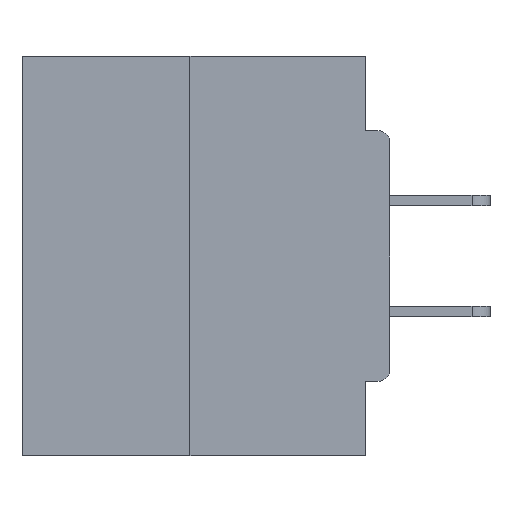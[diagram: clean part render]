
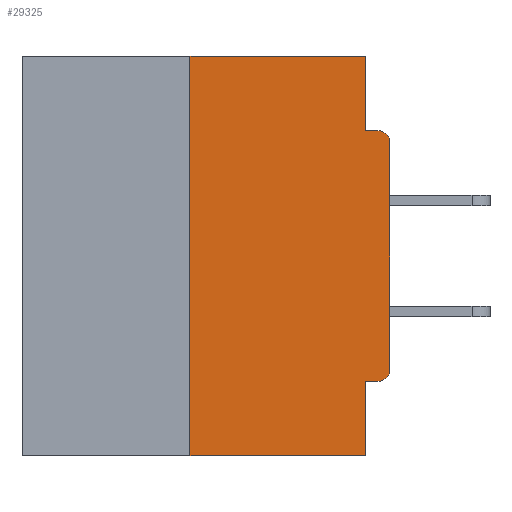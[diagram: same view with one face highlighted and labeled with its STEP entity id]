
A CAD part, left-side view. The second image highlights one B-rep face of the part: STEP entity #29325.
In plain terms, the highlighted planar face has unit normal (-1, 0, 0).
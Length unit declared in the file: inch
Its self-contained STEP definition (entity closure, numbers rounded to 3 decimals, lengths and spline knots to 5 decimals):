
#575 = LINE ( 'NONE', #21977, #9507 ) ;
#872 = CIRCLE ( 'NONE', #31588, 0.015 ) ;
#994 = CARTESIAN_POINT ( 'NONE',  ( 0., 0.46, 0. ) ) ;
#1197 = CARTESIAN_POINT ( 'NONE',  ( 0., 0.031, -0.0935 ) ) ;
#1281 = VECTOR ( 'NONE', #32515, 39.37008 ) ;
#1293 = CARTESIAN_POINT ( 'NONE',  ( 0., 0., -0.4065 ) ) ;
#1433 = DIRECTION ( 'NONE',  ( 0., -1., 0. ) ) ;
#2229 = LINE ( 'NONE', #38369, #1281 ) ;
#2484 = CARTESIAN_POINT ( 'NONE',  ( 0., 0., -0.3915 ) ) ;
#3401 = CARTESIAN_POINT ( 'NONE',  ( 0., 0.25, 0. ) ) ;
#3453 = VECTOR ( 'NONE', #20346, 39.37008 ) ;
#3644 = AXIS2_PLACEMENT_3D ( 'NONE', #15115, #14986, #6227 ) ;
#3993 = AXIS2_PLACEMENT_3D ( 'NONE', #36569, #6404, #12547 ) ;
#4587 = ORIENTED_EDGE ( 'NONE', *, *, #15984, .T. ) ;
#4954 = VECTOR ( 'NONE', #37236, 39.37008 ) ;
#5242 = DIRECTION ( 'NONE',  ( -1., 0., 0. ) ) ;
#6227 = DIRECTION ( 'NONE',  ( 0., 0., -1. ) ) ;
#6404 = DIRECTION ( 'NONE',  ( -1., 0., 0. ) ) ;
#7098 = VECTOR ( 'NONE', #31059, 39.37008 ) ;
#8372 = CARTESIAN_POINT ( 'NONE',  ( 0., 0.25, -0.5 ) ) ;
#8419 = VERTEX_POINT ( 'NONE', #30548 ) ;
#8903 = CARTESIAN_POINT ( 'NONE',  ( 0., 0.031, 0. ) ) ;
#9379 = EDGE_CURVE ( 'NONE', #21108, #22341, #33854, .T. ) ;
#9507 = VECTOR ( 'NONE', #12649, 39.37008 ) ;
#11661 = CARTESIAN_POINT ( 'NONE',  ( 0., 0.015, -0.1085 ) ) ;
#11968 = LINE ( 'NONE', #1293, #4954 ) ;
#12340 = LINE ( 'NONE', #22180, #3453 ) ;
#12547 = DIRECTION ( 'NONE',  ( 0., 0., -1. ) ) ;
#12649 = DIRECTION ( 'NONE',  ( 0., 0., 1. ) ) ;
#12778 = ORIENTED_EDGE ( 'NONE', *, *, #9379, .F. ) ;
#14009 = CARTESIAN_POINT ( 'NONE',  ( 0., 0., -0.1085 ) ) ;
#14609 = ORIENTED_EDGE ( 'NONE', *, *, #23510, .T. ) ;
#14707 = CARTESIAN_POINT ( 'NONE',  ( 0., 0.25, 0. ) ) ;
#14986 = DIRECTION ( 'NONE',  ( 1., 0., 0. ) ) ;
#15112 = ORIENTED_EDGE ( 'NONE', *, *, #18907, .F. ) ;
#15115 = CARTESIAN_POINT ( 'NONE',  ( 0., 0.46, 0. ) ) ;
#15802 = ORIENTED_EDGE ( 'NONE', *, *, #32103, .F. ) ;
#15984 = EDGE_CURVE ( 'NONE', #31399, #33786, #575, .T. ) ;
#16483 = VECTOR ( 'NONE', #29881, 39.37008 ) ;
#18907 = EDGE_CURVE ( 'NONE', #22341, #27713, #22138, .T. ) ;
#18994 = FACE_OUTER_BOUND ( 'NONE', #32371, .T. ) ;
#19898 = VERTEX_POINT ( 'NONE', #8372 ) ;
#20346 = DIRECTION ( 'NONE',  ( 0., -1., 0. ) ) ;
#20741 = CARTESIAN_POINT ( 'NONE',  ( 0., 0.031, -0.5 ) ) ;
#21108 = VERTEX_POINT ( 'NONE', #14707 ) ;
#21977 = CARTESIAN_POINT ( 'NONE',  ( 0., 0., 0. ) ) ;
#22138 = LINE ( 'NONE', #8903, #16483 ) ;
#22180 = CARTESIAN_POINT ( 'NONE',  ( 0., 0.46, -0.5 ) ) ;
#22264 = EDGE_CURVE ( 'NONE', #8419, #29533, #11968, .T. ) ;
#22341 = VERTEX_POINT ( 'NONE', #22963 ) ;
#22963 = CARTESIAN_POINT ( 'NONE',  ( 0., 0.031, 0. ) ) ;
#23116 = ORIENTED_EDGE ( 'NONE', *, *, #22264, .F. ) ;
#23510 = EDGE_CURVE ( 'NONE', #19898, #28562, #12340, .T. ) ;
#23683 = EDGE_CURVE ( 'NONE', #8419, #31399, #35816, .T. ) ;
#23765 = VECTOR ( 'NONE', #1433, 39.37008 ) ;
#23846 = PLANE ( 'NONE',  #3644 ) ;
#23884 = LINE ( 'NONE', #3401, #33725 ) ;
#24149 = DIRECTION ( 'NONE',  ( 0., 0., 1. ) ) ;
#25666 = VERTEX_POINT ( 'NONE', #35233 ) ;
#26091 = LINE ( 'NONE', #31517, #23765 ) ;
#26609 = ORIENTED_EDGE ( 'NONE', *, *, #23683, .T. ) ;
#27147 = ORIENTED_EDGE ( 'NONE', *, *, #36250, .F. ) ;
#27713 = VERTEX_POINT ( 'NONE', #1197 ) ;
#28266 = EDGE_CURVE ( 'NONE', #27713, #25666, #26091, .T. ) ;
#28562 = VERTEX_POINT ( 'NONE', #20741 ) ;
#29325 = ADVANCED_FACE ( 'NONE', ( #18994 ), #23846, .F. ) ;
#29533 = VERTEX_POINT ( 'NONE', #36394 ) ;
#29881 = DIRECTION ( 'NONE',  ( 0., 0., -1. ) ) ;
#30548 = CARTESIAN_POINT ( 'NONE',  ( 0., 0.015, -0.4065 ) ) ;
#31059 = DIRECTION ( 'NONE',  ( 0., -1., 0. ) ) ;
#31399 = VERTEX_POINT ( 'NONE', #2484 ) ;
#31470 = ORIENTED_EDGE ( 'NONE', *, *, #31498, .T. ) ;
#31498 = EDGE_CURVE ( 'NONE', #33786, #25666, #872, .T. ) ;
#31517 = CARTESIAN_POINT ( 'NONE',  ( 0., 0., -0.0935 ) ) ;
#31588 = AXIS2_PLACEMENT_3D ( 'NONE', #11661, #5242, #32689 ) ;
#32103 = EDGE_CURVE ( 'NONE', #29533, #28562, #2229, .T. ) ;
#32285 = ORIENTED_EDGE ( 'NONE', *, *, #28266, .F. ) ;
#32371 = EDGE_LOOP ( 'NONE', ( #12778, #27147, #14609, #15802, #23116, #26609, #4587, #31470, #32285, #15112 ) ) ;
#32515 = DIRECTION ( 'NONE',  ( 0., 0., -1. ) ) ;
#32689 = DIRECTION ( 'NONE',  ( 0., 0., -1. ) ) ;
#33725 = VECTOR ( 'NONE', #24149, 39.37008 ) ;
#33786 = VERTEX_POINT ( 'NONE', #14009 ) ;
#33854 = LINE ( 'NONE', #994, #7098 ) ;
#35233 = CARTESIAN_POINT ( 'NONE',  ( 0., 0.015, -0.0935 ) ) ;
#35816 = CIRCLE ( 'NONE', #3993, 0.015 ) ;
#36250 = EDGE_CURVE ( 'NONE', #19898, #21108, #23884, .T. ) ;
#36394 = CARTESIAN_POINT ( 'NONE',  ( 0., 0.031, -0.4065 ) ) ;
#36569 = CARTESIAN_POINT ( 'NONE',  ( 0., 0.015, -0.3915 ) ) ;
#37236 = DIRECTION ( 'NONE',  ( 0., 1., 0. ) ) ;
#38369 = CARTESIAN_POINT ( 'NONE',  ( 0., 0.031, -0.5 ) ) ;
